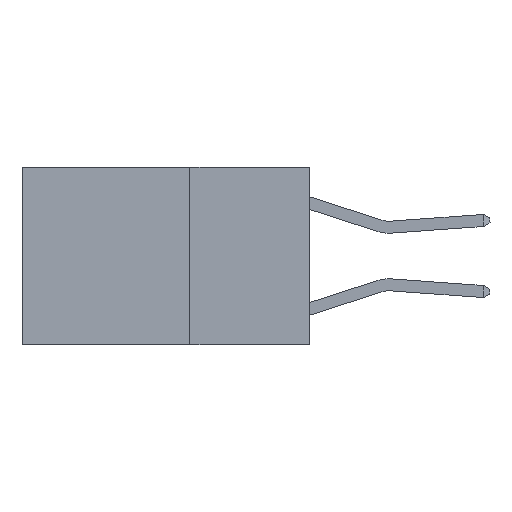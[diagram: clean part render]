
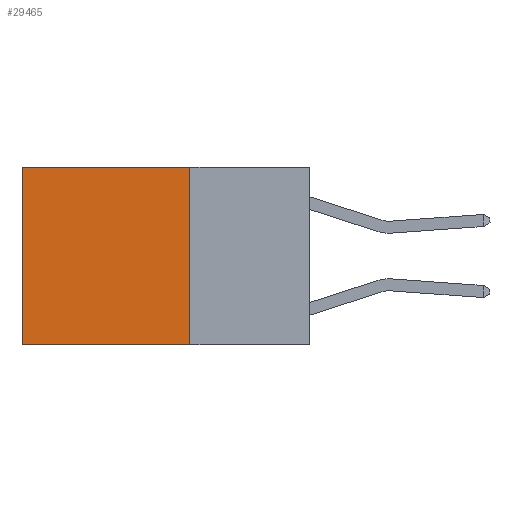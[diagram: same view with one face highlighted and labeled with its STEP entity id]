
A CAD part, left-side view. The second image highlights one B-rep face of the part: STEP entity #29465.
In plain terms, the highlighted planar face has unit normal (-1, 0, 0).
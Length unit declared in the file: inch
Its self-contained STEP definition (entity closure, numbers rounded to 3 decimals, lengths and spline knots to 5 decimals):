
#470 = CARTESIAN_POINT ( 'NONE',  ( 0.2625, 0.25, 0. ) ) ;
#1263 = EDGE_CURVE ( 'NONE', #15039, #22147, #24160, .T. ) ;
#2377 = DIRECTION ( 'NONE',  ( 0., 1., 0. ) ) ;
#2582 = VERTEX_POINT ( 'NONE', #470 ) ;
#2792 = LINE ( 'NONE', #13324, #15119 ) ;
#2940 = ORIENTED_EDGE ( 'NONE', *, *, #17644, .T. ) ;
#3197 = CARTESIAN_POINT ( 'NONE',  ( 0.2625, 0.6, -0.37 ) ) ;
#4157 = LINE ( 'NONE', #20165, #28937 ) ;
#4992 = DIRECTION ( 'NONE',  ( 0., 0., -1. ) ) ;
#5338 = ORIENTED_EDGE ( 'NONE', *, *, #25238, .F. ) ;
#5564 = DIRECTION ( 'NONE',  ( 0., 0., -1. ) ) ;
#6219 = DIRECTION ( 'NONE',  ( 0., 1., 0. ) ) ;
#9258 = CARTESIAN_POINT ( 'NONE',  ( 0.2625, 0.25, -0.37 ) ) ;
#11649 = ORIENTED_EDGE ( 'NONE', *, *, #17847, .F. ) ;
#12976 = EDGE_LOOP ( 'NONE', ( #27182, #11649, #5338, #2940 ) ) ;
#13324 = CARTESIAN_POINT ( 'NONE',  ( 0.2625, 0.25, 0. ) ) ;
#14227 = CARTESIAN_POINT ( 'NONE',  ( 0.2625, 0.6, 0. ) ) ;
#15025 = VECTOR ( 'NONE', #2377, 39.37008 ) ;
#15039 = VERTEX_POINT ( 'NONE', #16196 ) ;
#15119 = VECTOR ( 'NONE', #15655, 39.37008 ) ;
#15655 = DIRECTION ( 'NONE',  ( 0., 0., -1. ) ) ;
#16196 = CARTESIAN_POINT ( 'NONE',  ( 0.2625, 0.6, 0. ) ) ;
#16469 = CARTESIAN_POINT ( 'NONE',  ( 0.2625, 0.25, -0.37 ) ) ;
#17138 = CARTESIAN_POINT ( 'NONE',  ( 0.2625, 0.25, 0. ) ) ;
#17644 = EDGE_CURVE ( 'NONE', #2582, #15039, #4157, .T. ) ;
#17847 = EDGE_CURVE ( 'NONE', #17923, #22147, #27451, .T. ) ;
#17923 = VERTEX_POINT ( 'NONE', #16469 ) ;
#19399 = PLANE ( 'NONE',  #29011 ) ;
#19500 = DIRECTION ( 'NONE',  ( 1., 0., 0. ) ) ;
#20165 = CARTESIAN_POINT ( 'NONE',  ( 0.2625, 0.25, 0. ) ) ;
#22147 = VERTEX_POINT ( 'NONE', #3197 ) ;
#24160 = LINE ( 'NONE', #14227, #29638 ) ;
#25238 = EDGE_CURVE ( 'NONE', #2582, #17923, #2792, .T. ) ;
#27182 = ORIENTED_EDGE ( 'NONE', *, *, #1263, .T. ) ;
#27451 = LINE ( 'NONE', #9258, #15025 ) ;
#27761 = FACE_OUTER_BOUND ( 'NONE', #12976, .T. ) ;
#28937 = VECTOR ( 'NONE', #6219, 39.37008 ) ;
#29011 = AXIS2_PLACEMENT_3D ( 'NONE', #17138, #19500, #5564 ) ;
#29465 = ADVANCED_FACE ( 'NONE', ( #27761 ), #19399, .F. ) ;
#29638 = VECTOR ( 'NONE', #4992, 39.37008 ) ;
